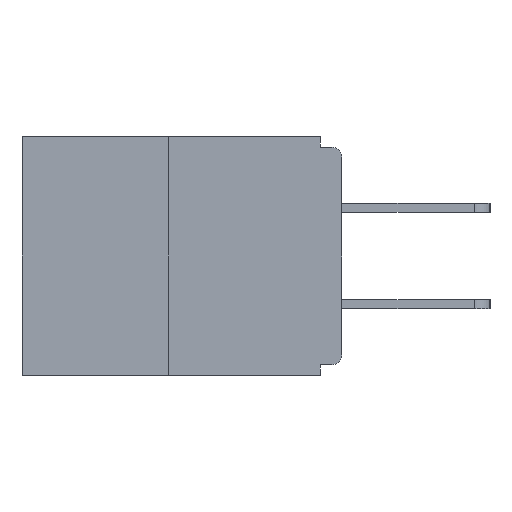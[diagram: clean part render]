
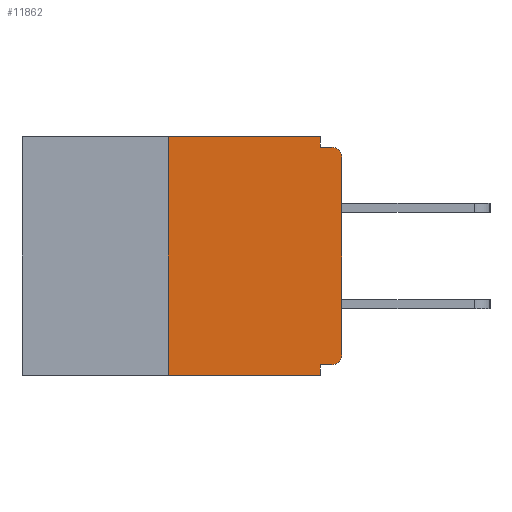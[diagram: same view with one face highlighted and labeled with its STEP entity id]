
A CAD part, left-side view. The second image highlights one B-rep face of the part: STEP entity #11862.
In plain terms, the highlighted planar face has unit normal (-1, 0, 0).
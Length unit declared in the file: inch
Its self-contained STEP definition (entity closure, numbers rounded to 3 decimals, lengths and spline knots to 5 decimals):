
#91 = CIRCLE ( 'NONE', #21193, 0.015 ) ;
#297 = CARTESIAN_POINT ( 'NONE',  ( 0., 0.031, -0.343 ) ) ;
#420 = DIRECTION ( 'NONE',  ( 0., 0., 1. ) ) ;
#452 = DIRECTION ( 'NONE',  ( -1., 0., 0. ) ) ;
#454 = VECTOR ( 'NONE', #2516, 39.37008 ) ;
#878 = CARTESIAN_POINT ( 'NONE',  ( 0., 0., -0.313 ) ) ;
#924 = VERTEX_POINT ( 'NONE', #9914 ) ;
#1082 = EDGE_CURVE ( 'NONE', #8141, #17468, #19654, .T. ) ;
#1164 = VECTOR ( 'NONE', #6784, 39.37008 ) ;
#1569 = VECTOR ( 'NONE', #8207, 39.37008 ) ;
#2516 = DIRECTION ( 'NONE',  ( 0., 1., 0. ) ) ;
#2675 = ORIENTED_EDGE ( 'NONE', *, *, #19984, .F. ) ;
#2750 = LINE ( 'NONE', #9470, #19760 ) ;
#3020 = ORIENTED_EDGE ( 'NONE', *, *, #6679, .T. ) ;
#3596 = CARTESIAN_POINT ( 'NONE',  ( 0., 0.031, -0.343 ) ) ;
#4054 = CARTESIAN_POINT ( 'NONE',  ( 0., 0., -0.328 ) ) ;
#4093 = VERTEX_POINT ( 'NONE', #878 ) ;
#4102 = CARTESIAN_POINT ( 'NONE',  ( 0., 0.031, -0.328 ) ) ;
#4284 = DIRECTION ( 'NONE',  ( 0., 0., -1. ) ) ;
#4406 = EDGE_CURVE ( 'NONE', #924, #17468, #8656, .T. ) ;
#4555 = CARTESIAN_POINT ( 'NONE',  ( 0., 0.46, 0. ) ) ;
#4569 = AXIS2_PLACEMENT_3D ( 'NONE', #4555, #18065, #4668 ) ;
#4668 = DIRECTION ( 'NONE',  ( 0., 0., -1. ) ) ;
#4879 = CARTESIAN_POINT ( 'NONE',  ( 0., 0.031, 0. ) ) ;
#5369 = VECTOR ( 'NONE', #14153, 39.37008 ) ;
#5767 = CARTESIAN_POINT ( 'NONE',  ( 0., 0.25, -0.343 ) ) ;
#5842 = VERTEX_POINT ( 'NONE', #297 ) ;
#6191 = ORIENTED_EDGE ( 'NONE', *, *, #8036, .F. ) ;
#6638 = CARTESIAN_POINT ( 'NONE',  ( 0., 0.031, 0. ) ) ;
#6676 = LINE ( 'NONE', #3596, #1164 ) ;
#6679 = EDGE_CURVE ( 'NONE', #16839, #5842, #9757, .T. ) ;
#6784 = DIRECTION ( 'NONE',  ( 0., 0., -1. ) ) ;
#6789 = CARTESIAN_POINT ( 'NONE',  ( 0., 0.015, -0.328 ) ) ;
#6811 = VERTEX_POINT ( 'NONE', #6638 ) ;
#7609 = CARTESIAN_POINT ( 'NONE',  ( 0., 0.015, -0.313 ) ) ;
#7678 = EDGE_CURVE ( 'NONE', #16839, #17905, #12325, .T. ) ;
#7739 = CARTESIAN_POINT ( 'NONE',  ( 0., 0.015, -0.015 ) ) ;
#8008 = VECTOR ( 'NONE', #420, 39.37008 ) ;
#8036 = EDGE_CURVE ( 'NONE', #17375, #5842, #6676, .T. ) ;
#8141 = VERTEX_POINT ( 'NONE', #17750 ) ;
#8207 = DIRECTION ( 'NONE',  ( 0., 0., -1. ) ) ;
#8214 = CARTESIAN_POINT ( 'NONE',  ( 0., 0.46, -0.343 ) ) ;
#8656 = LINE ( 'NONE', #20348, #20599 ) ;
#8806 = DIRECTION ( 'NONE',  ( 0., 0., -1. ) ) ;
#9470 = CARTESIAN_POINT ( 'NONE',  ( 0., 0., 0. ) ) ;
#9757 = LINE ( 'NONE', #8214, #16689 ) ;
#9914 = CARTESIAN_POINT ( 'NONE',  ( 0., 0.031, -0.015 ) ) ;
#10126 = AXIS2_PLACEMENT_3D ( 'NONE', #20725, #452, #8806 ) ;
#10171 = ORIENTED_EDGE ( 'NONE', *, *, #4406, .F. ) ;
#11269 = ORIENTED_EDGE ( 'NONE', *, *, #15431, .F. ) ;
#11365 = DIRECTION ( 'NONE',  ( 0., 0., 1. ) ) ;
#11862 = ADVANCED_FACE ( 'NONE', ( #12994 ), #19701, .F. ) ;
#12062 = ORIENTED_EDGE ( 'NONE', *, *, #7678, .F. ) ;
#12325 = LINE ( 'NONE', #17082, #8008 ) ;
#12466 = EDGE_CURVE ( 'NONE', #4093, #8141, #2750, .T. ) ;
#12994 = FACE_OUTER_BOUND ( 'NONE', #15483, .T. ) ;
#13456 = ORIENTED_EDGE ( 'NONE', *, *, #12466, .T. ) ;
#13839 = CARTESIAN_POINT ( 'NONE',  ( 0., 0.46, 0. ) ) ;
#14013 = LINE ( 'NONE', #4054, #454 ) ;
#14153 = DIRECTION ( 'NONE',  ( 0., -1., 0. ) ) ;
#14360 = DIRECTION ( 'NONE',  ( -1., 0., 0. ) ) ;
#15431 = EDGE_CURVE ( 'NONE', #16745, #17375, #14013, .T. ) ;
#15483 = EDGE_LOOP ( 'NONE', ( #18860, #12062, #3020, #6191, #11269, #15590, #13456, #18458, #10171, #2675 ) ) ;
#15590 = ORIENTED_EDGE ( 'NONE', *, *, #17829, .T. ) ;
#15976 = EDGE_CURVE ( 'NONE', #17905, #6811, #20760, .T. ) ;
#16406 = DIRECTION ( 'NONE',  ( 0., -1., 0. ) ) ;
#16689 = VECTOR ( 'NONE', #16406, 39.37008 ) ;
#16745 = VERTEX_POINT ( 'NONE', #6789 ) ;
#16839 = VERTEX_POINT ( 'NONE', #5767 ) ;
#17082 = CARTESIAN_POINT ( 'NONE',  ( 0., 0.25, 0. ) ) ;
#17375 = VERTEX_POINT ( 'NONE', #4102 ) ;
#17468 = VERTEX_POINT ( 'NONE', #7739 ) ;
#17748 = CARTESIAN_POINT ( 'NONE',  ( 0., 0.25, 0. ) ) ;
#17750 = CARTESIAN_POINT ( 'NONE',  ( 0., 0., -0.03 ) ) ;
#17829 = EDGE_CURVE ( 'NONE', #16745, #4093, #91, .T. ) ;
#17905 = VERTEX_POINT ( 'NONE', #17748 ) ;
#18065 = DIRECTION ( 'NONE',  ( 1., 0., 0. ) ) ;
#18458 = ORIENTED_EDGE ( 'NONE', *, *, #1082, .T. ) ;
#18797 = DIRECTION ( 'NONE',  ( 0., -1., 0. ) ) ;
#18860 = ORIENTED_EDGE ( 'NONE', *, *, #15976, .F. ) ;
#19654 = CIRCLE ( 'NONE', #10126, 0.015 ) ;
#19701 = PLANE ( 'NONE',  #4569 ) ;
#19760 = VECTOR ( 'NONE', #11365, 39.37008 ) ;
#19984 = EDGE_CURVE ( 'NONE', #6811, #924, #20025, .T. ) ;
#20025 = LINE ( 'NONE', #4879, #1569 ) ;
#20348 = CARTESIAN_POINT ( 'NONE',  ( 0., 0., -0.015 ) ) ;
#20599 = VECTOR ( 'NONE', #18797, 39.37008 ) ;
#20725 = CARTESIAN_POINT ( 'NONE',  ( 0., 0.015, -0.03 ) ) ;
#20760 = LINE ( 'NONE', #13839, #5369 ) ;
#21193 = AXIS2_PLACEMENT_3D ( 'NONE', #7609, #14360, #4284 ) ;
